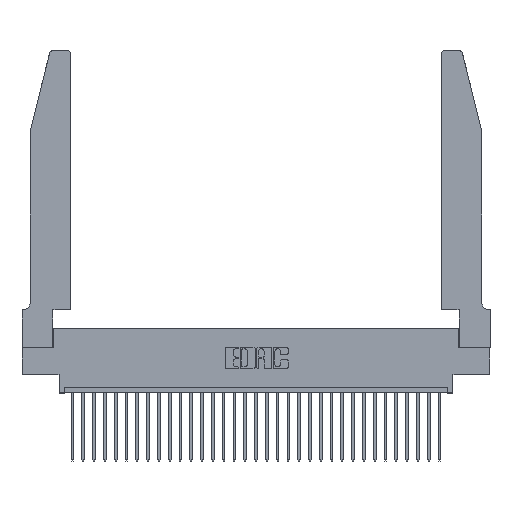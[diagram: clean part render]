
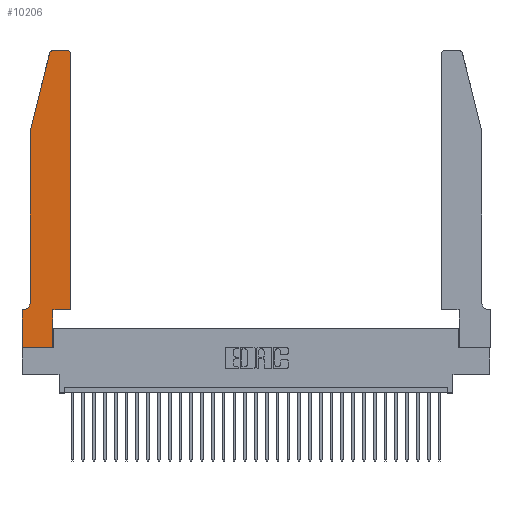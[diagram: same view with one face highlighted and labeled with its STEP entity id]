
A CAD part, top view. The second image highlights one B-rep face of the part: STEP entity #10206.
In plain terms, the highlighted planar face has unit normal (0, 0, 1).
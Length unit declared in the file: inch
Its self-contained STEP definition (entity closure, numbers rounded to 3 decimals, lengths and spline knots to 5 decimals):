
#871 = VERTEX_POINT ( 'NONE', #18217 ) ;
#1290 = EDGE_CURVE ( 'NONE', #30644, #22452, #28151, .T. ) ;
#1754 = DIRECTION ( 'NONE',  ( 0., 0., 1. ) ) ;
#1790 = ORIENTED_EDGE ( 'NONE', *, *, #22984, .T. ) ;
#2074 = VECTOR ( 'NONE', #10875, 39.37008 ) ;
#2122 = VECTOR ( 'NONE', #10460, 39.37008 ) ;
#2177 = VERTEX_POINT ( 'NONE', #4242 ) ;
#2322 = LINE ( 'NONE', #26557, #20986 ) ;
#2501 = LINE ( 'NONE', #20652, #2122 ) ;
#2600 = DIRECTION ( 'NONE',  ( -1., 0., 0. ) ) ;
#2704 = CARTESIAN_POINT ( 'NONE',  ( 0., 0.35, 0.37 ) ) ;
#2752 = ORIENTED_EDGE ( 'NONE', *, *, #1290, .T. ) ;
#3071 = CARTESIAN_POINT ( 'NONE',  ( 0.284, 2.75, 0.37 ) ) ;
#3560 = CARTESIAN_POINT ( 'NONE',  ( 0.4205, 2.75, 0.37 ) ) ;
#4011 = AXIS2_PLACEMENT_3D ( 'NONE', #19387, #9610, #11911 ) ;
#4242 = CARTESIAN_POINT ( 'NONE',  ( 0.2865, 0., 0.37 ) ) ;
#4477 = VECTOR ( 'NONE', #25437, 39.37008 ) ;
#4627 = AXIS2_PLACEMENT_3D ( 'NONE', #29482, #9823, #11897 ) ;
#5004 = EDGE_CURVE ( 'NONE', #6993, #7352, #26786, .T. ) ;
#5072 = CARTESIAN_POINT ( 'NONE',  ( 0.25487, 2.72718, 0.37 ) ) ;
#5734 = CARTESIAN_POINT ( 'NONE',  ( 0., 0., 0.37 ) ) ;
#5771 = ORIENTED_EDGE ( 'NONE', *, *, #16284, .T. ) ;
#6849 = CIRCLE ( 'NONE', #21382, 0.03 ) ;
#6850 = CARTESIAN_POINT ( 'NONE',  ( 0.0755, 2., 0.37 ) ) ;
#6914 = VERTEX_POINT ( 'NONE', #5072 ) ;
#6969 = LINE ( 'NONE', #6850, #31816 ) ;
#6993 = VERTEX_POINT ( 'NONE', #19678 ) ;
#7108 = CARTESIAN_POINT ( 'NONE',  ( 0., 0.35, 0.37 ) ) ;
#7352 = VERTEX_POINT ( 'NONE', #12258 ) ;
#8432 = LINE ( 'NONE', #19410, #20897 ) ;
#9387 = DIRECTION ( 'NONE',  ( 0., -1., 0. ) ) ;
#9597 = ORIENTED_EDGE ( 'NONE', *, *, #27311, .T. ) ;
#9610 = DIRECTION ( 'NONE',  ( 0., 0., 1. ) ) ;
#9823 = DIRECTION ( 'NONE',  ( 0., 0., -1. ) ) ;
#10206 = ADVANCED_FACE ( 'NONE', ( #20438 ), #22002, .T. ) ;
#10440 = ORIENTED_EDGE ( 'NONE', *, *, #15174, .T. ) ;
#10460 = DIRECTION ( 'NONE',  ( -0.239, -0.971, 0. ) ) ;
#10875 = DIRECTION ( 'NONE',  ( 1., 0., 0. ) ) ;
#11124 = CARTESIAN_POINT ( 'NONE',  ( 0.4505, 2.72, 0.37 ) ) ;
#11162 = VERTEX_POINT ( 'NONE', #11124 ) ;
#11347 = VECTOR ( 'NONE', #2600, 39.37008 ) ;
#11678 = VERTEX_POINT ( 'NONE', #3071 ) ;
#11897 = DIRECTION ( 'NONE',  ( -1., 0., 0. ) ) ;
#11911 = DIRECTION ( 'NONE',  ( 1., 0., 0. ) ) ;
#12258 = CARTESIAN_POINT ( 'NONE',  ( 0.0055, 0.35, 0.37 ) ) ;
#13190 = LINE ( 'NONE', #20012, #32174 ) ;
#13570 = DIRECTION ( 'NONE',  ( 1., 0., 0. ) ) ;
#14234 = ORIENTED_EDGE ( 'NONE', *, *, #24496, .T. ) ;
#14452 = ORIENTED_EDGE ( 'NONE', *, *, #25219, .T. ) ;
#14607 = ORIENTED_EDGE ( 'NONE', *, *, #17643, .T. ) ;
#14799 = VERTEX_POINT ( 'NONE', #3560 ) ;
#15174 = EDGE_CURVE ( 'NONE', #11678, #6914, #6849, .T. ) ;
#15261 = CARTESIAN_POINT ( 'NONE',  ( 0.2865, 0.35, 0.37 ) ) ;
#16284 = EDGE_CURVE ( 'NONE', #6914, #31234, #2501, .T. ) ;
#17643 = EDGE_CURVE ( 'NONE', #7352, #30644, #26508, .T. ) ;
#17658 = VECTOR ( 'NONE', #29099, 39.37008 ) ;
#17914 = CARTESIAN_POINT ( 'NONE',  ( 0.0755, 2., 0.37 ) ) ;
#17946 = CARTESIAN_POINT ( 'NONE',  ( 0.2605, 2.75, 0.37 ) ) ;
#18217 = CARTESIAN_POINT ( 'NONE',  ( 0.4505, 0.35, 0.37 ) ) ;
#19111 = LINE ( 'NONE', #17946, #11347 ) ;
#19387 = CARTESIAN_POINT ( 'NONE',  ( 0.4205, 2.72, 0.37 ) ) ;
#19410 = CARTESIAN_POINT ( 'NONE',  ( 0., 0., 0.37 ) ) ;
#19678 = CARTESIAN_POINT ( 'NONE',  ( 0.0755, 0.42, 0.37 ) ) ;
#20012 = CARTESIAN_POINT ( 'NONE',  ( 0.4505, 0.35, 0.37 ) ) ;
#20438 = FACE_OUTER_BOUND ( 'NONE', #30732, .T. ) ;
#20652 = CARTESIAN_POINT ( 'NONE',  ( 0.0755, 2., 0.37 ) ) ;
#20754 = CARTESIAN_POINT ( 'NONE',  ( 0.4505, 0.35, 0.37 ) ) ;
#20897 = VECTOR ( 'NONE', #13570, 39.37008 ) ;
#20986 = VECTOR ( 'NONE', #29368, 39.37008 ) ;
#21382 = AXIS2_PLACEMENT_3D ( 'NONE', #25684, #27723, #25265 ) ;
#21445 = EDGE_CURVE ( 'NONE', #25714, #871, #23054, .T. ) ;
#21609 = ORIENTED_EDGE ( 'NONE', *, *, #26042, .T. ) ;
#22002 = PLANE ( 'NONE',  #23262 ) ;
#22452 = VERTEX_POINT ( 'NONE', #5734 ) ;
#22659 = CARTESIAN_POINT ( 'NONE',  ( 0.0755, 0.35, 0.37 ) ) ;
#22984 = EDGE_CURVE ( 'NONE', #11162, #14799, #25641, .T. ) ;
#23054 = LINE ( 'NONE', #20754, #2074 ) ;
#23262 = AXIS2_PLACEMENT_3D ( 'NONE', #7108, #1754, #24470 ) ;
#23538 = EDGE_CURVE ( 'NONE', #31234, #6993, #6969, .T. ) ;
#24470 = DIRECTION ( 'NONE',  ( 1., 0., 0. ) ) ;
#24496 = EDGE_CURVE ( 'NONE', #871, #11162, #13190, .T. ) ;
#25219 = EDGE_CURVE ( 'NONE', #14799, #11678, #19111, .T. ) ;
#25265 = DIRECTION ( 'NONE',  ( 1., 0., 0. ) ) ;
#25437 = DIRECTION ( 'NONE',  ( 0., -1., 0. ) ) ;
#25641 = CIRCLE ( 'NONE', #4011, 0.03 ) ;
#25684 = CARTESIAN_POINT ( 'NONE',  ( 0.284, 2.72, 0.37 ) ) ;
#25714 = VERTEX_POINT ( 'NONE', #15261 ) ;
#26042 = EDGE_CURVE ( 'NONE', #2177, #25714, #2322, .T. ) ;
#26508 = LINE ( 'NONE', #22659, #17658 ) ;
#26557 = CARTESIAN_POINT ( 'NONE',  ( 0.2865, 0.35, 0.37 ) ) ;
#26786 = CIRCLE ( 'NONE', #4627, 0.07 ) ;
#27311 = EDGE_CURVE ( 'NONE', #22452, #2177, #8432, .T. ) ;
#27723 = DIRECTION ( 'NONE',  ( 0., 0., 1. ) ) ;
#28151 = LINE ( 'NONE', #29978, #4477 ) ;
#29099 = DIRECTION ( 'NONE',  ( -1., 0., 0. ) ) ;
#29368 = DIRECTION ( 'NONE',  ( 0., 1., 0. ) ) ;
#29482 = CARTESIAN_POINT ( 'NONE',  ( 0.0055, 0.42, 0.37 ) ) ;
#29483 = DIRECTION ( 'NONE',  ( 0., 1., 0. ) ) ;
#29547 = ORIENTED_EDGE ( 'NONE', *, *, #23538, .T. ) ;
#29978 = CARTESIAN_POINT ( 'NONE',  ( 0., 0., 0.37 ) ) ;
#30475 = ORIENTED_EDGE ( 'NONE', *, *, #21445, .T. ) ;
#30644 = VERTEX_POINT ( 'NONE', #2704 ) ;
#30732 = EDGE_LOOP ( 'NONE', ( #14452, #10440, #5771, #29547, #32003, #14607, #2752, #9597, #21609, #30475, #14234, #1790 ) ) ;
#31234 = VERTEX_POINT ( 'NONE', #17914 ) ;
#31816 = VECTOR ( 'NONE', #9387, 39.37008 ) ;
#32003 = ORIENTED_EDGE ( 'NONE', *, *, #5004, .T. ) ;
#32174 = VECTOR ( 'NONE', #29483, 39.37008 ) ;
